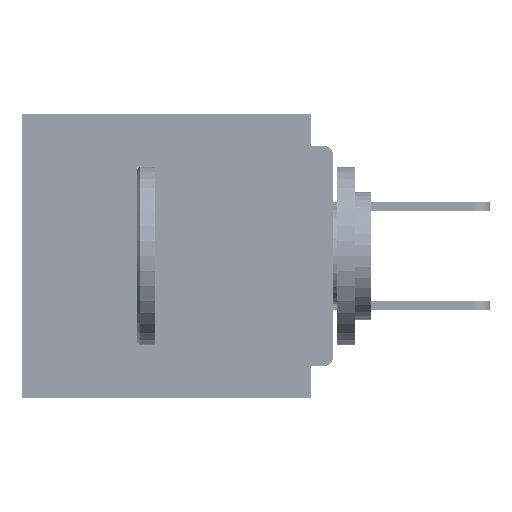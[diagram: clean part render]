
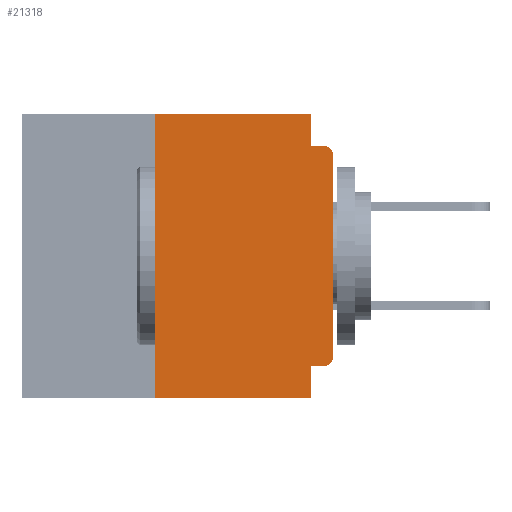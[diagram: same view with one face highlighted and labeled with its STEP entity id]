
A CAD part, left-side view. The second image highlights one B-rep face of the part: STEP entity #21318.
In plain terms, the highlighted planar face has unit normal (-1, 0, 0).
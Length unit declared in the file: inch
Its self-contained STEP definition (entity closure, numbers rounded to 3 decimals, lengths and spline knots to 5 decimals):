
#290 = CARTESIAN_POINT ( 'NONE',  ( 0., 0.031, -0.4 ) ) ;
#362 = CIRCLE ( 'NONE', #37082, 0.015 ) ;
#688 = VERTEX_POINT ( 'NONE', #64760 ) ;
#1867 = ORIENTED_EDGE ( 'NONE', *, *, #27844, .F. ) ;
#2848 = VERTEX_POINT ( 'NONE', #32647 ) ;
#3145 = DIRECTION ( 'NONE',  ( 0., 1., 0. ) ) ;
#3195 = VECTOR ( 'NONE', #23269, 39.37008 ) ;
#3462 = LINE ( 'NONE', #39470, #14055 ) ;
#3634 = VECTOR ( 'NONE', #26144, 39.37008 ) ;
#4016 = VERTEX_POINT ( 'NONE', #36330 ) ;
#4299 = CIRCLE ( 'NONE', #43932, 0.015 ) ;
#4406 = CARTESIAN_POINT ( 'NONE',  ( 0., 0.437, 0. ) ) ;
#5097 = VECTOR ( 'NONE', #13326, 39.37008 ) ;
#5975 = CARTESIAN_POINT ( 'NONE',  ( 0., 0., -0.06 ) ) ;
#7781 = ORIENTED_EDGE ( 'NONE', *, *, #17273, .F. ) ;
#8005 = ORIENTED_EDGE ( 'NONE', *, *, #41953, .T. ) ;
#9376 = LINE ( 'NONE', #21653, #21544 ) ;
#13326 = DIRECTION ( 'NONE',  ( 0., 0., -1. ) ) ;
#13689 = EDGE_CURVE ( 'NONE', #45161, #60234, #30852, .T. ) ;
#14055 = VECTOR ( 'NONE', #44734, 39.37008 ) ;
#14395 = CARTESIAN_POINT ( 'NONE',  ( 0., 0.031, 0. ) ) ;
#15284 = EDGE_CURVE ( 'NONE', #25724, #45161, #29786, .T. ) ;
#15336 = VECTOR ( 'NONE', #3145, 39.37008 ) ;
#15845 = ORIENTED_EDGE ( 'NONE', *, *, #37818, .T. ) ;
#16951 = LINE ( 'NONE', #44698, #15336 ) ;
#17111 = ORIENTED_EDGE ( 'NONE', *, *, #20533, .F. ) ;
#17273 = EDGE_CURVE ( 'NONE', #60234, #43992, #32745, .T. ) ;
#18487 = ORIENTED_EDGE ( 'NONE', *, *, #64976, .T. ) ;
#20533 = EDGE_CURVE ( 'NONE', #4016, #46485, #16951, .T. ) ;
#21300 = CARTESIAN_POINT ( 'NONE',  ( 0., 0.015, -0.06 ) ) ;
#21318 = ADVANCED_FACE ( 'NONE', ( #33181 ), #35512, .F. ) ;
#21544 = VECTOR ( 'NONE', #26885, 39.37008 ) ;
#21653 = CARTESIAN_POINT ( 'NONE',  ( 0., 0., 0. ) ) ;
#22489 = CARTESIAN_POINT ( 'NONE',  ( 0., 0.031, -0.355 ) ) ;
#22611 = ORIENTED_EDGE ( 'NONE', *, *, #13689, .F. ) ;
#23269 = DIRECTION ( 'NONE',  ( 0., -1., 0. ) ) ;
#23697 = VERTEX_POINT ( 'NONE', #50636 ) ;
#24672 = LINE ( 'NONE', #29046, #36870 ) ;
#25724 = VERTEX_POINT ( 'NONE', #57580 ) ;
#26144 = DIRECTION ( 'NONE',  ( 0., 0., -1. ) ) ;
#26301 = ORIENTED_EDGE ( 'NONE', *, *, #38051, .F. ) ;
#26533 = DIRECTION ( 'NONE',  ( 0., 0., -1. ) ) ;
#26885 = DIRECTION ( 'NONE',  ( 0., 0., 1. ) ) ;
#27059 = CARTESIAN_POINT ( 'NONE',  ( 0., 0.015, -0.34 ) ) ;
#27844 = EDGE_CURVE ( 'NONE', #46485, #2848, #45074, .T. ) ;
#28522 = CARTESIAN_POINT ( 'NONE',  ( 0., 0.437, 0. ) ) ;
#29046 = CARTESIAN_POINT ( 'NONE',  ( 0., 0.437, -0.4 ) ) ;
#29786 = LINE ( 'NONE', #53288, #55689 ) ;
#30852 = LINE ( 'NONE', #28522, #3195 ) ;
#32300 = DIRECTION ( 'NONE',  ( 0., 0., -1. ) ) ;
#32647 = CARTESIAN_POINT ( 'NONE',  ( 0., 0.031, -0.4 ) ) ;
#32745 = LINE ( 'NONE', #54796, #5097 ) ;
#32911 = DIRECTION ( 'NONE',  ( 0., 0., 1. ) ) ;
#33181 = FACE_OUTER_BOUND ( 'NONE', #55566, .T. ) ;
#35420 = CARTESIAN_POINT ( 'NONE',  ( 0., 0.031, -0.045 ) ) ;
#35512 = PLANE ( 'NONE',  #54092 ) ;
#35736 = DIRECTION ( 'NONE',  ( 0., 0., -1. ) ) ;
#36330 = CARTESIAN_POINT ( 'NONE',  ( 0., 0.015, -0.355 ) ) ;
#36870 = VECTOR ( 'NONE', #54853, 39.37008 ) ;
#37082 = AXIS2_PLACEMENT_3D ( 'NONE', #21300, #57547, #26533 ) ;
#37818 = EDGE_CURVE ( 'NONE', #4016, #23697, #4299, .T. ) ;
#38051 = EDGE_CURVE ( 'NONE', #43992, #688, #3462, .T. ) ;
#39470 = CARTESIAN_POINT ( 'NONE',  ( 0., 0., -0.045 ) ) ;
#40026 = CARTESIAN_POINT ( 'NONE',  ( 0., 0.25, 0. ) ) ;
#41905 = ORIENTED_EDGE ( 'NONE', *, *, #42827, .T. ) ;
#41953 = EDGE_CURVE ( 'NONE', #23697, #58030, #9376, .T. ) ;
#42827 = EDGE_CURVE ( 'NONE', #25724, #2848, #24672, .T. ) ;
#43932 = AXIS2_PLACEMENT_3D ( 'NONE', #27059, #63186, #32300 ) ;
#43992 = VERTEX_POINT ( 'NONE', #35420 ) ;
#44698 = CARTESIAN_POINT ( 'NONE',  ( 0., 0., -0.355 ) ) ;
#44734 = DIRECTION ( 'NONE',  ( 0., -1., 0. ) ) ;
#45074 = LINE ( 'NONE', #290, #3634 ) ;
#45161 = VERTEX_POINT ( 'NONE', #40026 ) ;
#46485 = VERTEX_POINT ( 'NONE', #22489 ) ;
#50636 = CARTESIAN_POINT ( 'NONE',  ( 0., 0., -0.34 ) ) ;
#53288 = CARTESIAN_POINT ( 'NONE',  ( 0., 0.25, -0.4 ) ) ;
#53495 = ORIENTED_EDGE ( 'NONE', *, *, #15284, .F. ) ;
#54092 = AXIS2_PLACEMENT_3D ( 'NONE', #4406, #66549, #35736 ) ;
#54796 = CARTESIAN_POINT ( 'NONE',  ( 0., 0.031, 0. ) ) ;
#54853 = DIRECTION ( 'NONE',  ( 0., -1., 0. ) ) ;
#55566 = EDGE_LOOP ( 'NONE', ( #8005, #18487, #26301, #7781, #22611, #53495, #41905, #1867, #17111, #15845 ) ) ;
#55689 = VECTOR ( 'NONE', #32911, 39.37008 ) ;
#57547 = DIRECTION ( 'NONE',  ( -1., 0., 0. ) ) ;
#57580 = CARTESIAN_POINT ( 'NONE',  ( 0., 0.25, -0.4 ) ) ;
#58030 = VERTEX_POINT ( 'NONE', #5975 ) ;
#60234 = VERTEX_POINT ( 'NONE', #14395 ) ;
#63186 = DIRECTION ( 'NONE',  ( -1., 0., 0. ) ) ;
#64760 = CARTESIAN_POINT ( 'NONE',  ( 0., 0.015, -0.045 ) ) ;
#64976 = EDGE_CURVE ( 'NONE', #58030, #688, #362, .T. ) ;
#66549 = DIRECTION ( 'NONE',  ( 1., 0., 0. ) ) ;
